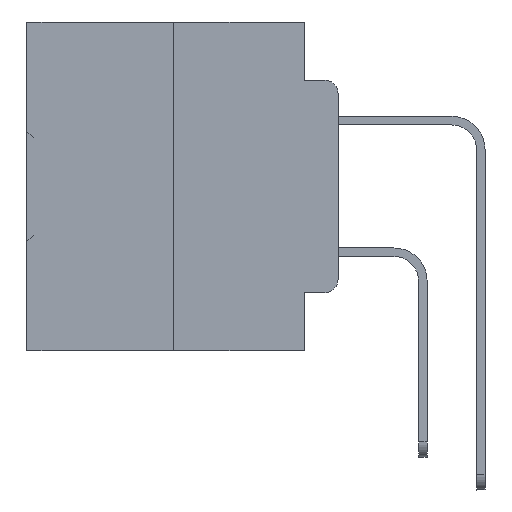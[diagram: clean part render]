
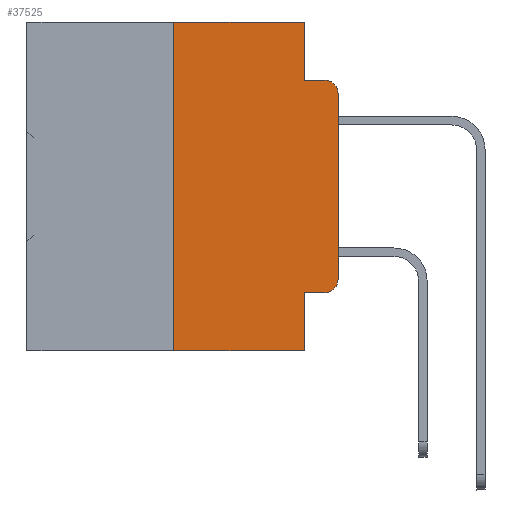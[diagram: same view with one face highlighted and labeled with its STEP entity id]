
A CAD part, left-side view. The second image highlights one B-rep face of the part: STEP entity #37525.
In plain terms, the highlighted planar face has unit normal (-1, 0, 0).
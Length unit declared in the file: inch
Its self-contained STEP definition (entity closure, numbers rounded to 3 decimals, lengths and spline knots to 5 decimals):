
#117 = CARTESIAN_POINT ( 'NONE',  ( 0., 0., 0. ) ) ;
#535 = VECTOR ( 'NONE', #15275, 39.37008 ) ;
#956 = LINE ( 'NONE', #13069, #31611 ) ;
#3079 = EDGE_CURVE ( 'NONE', #16572, #5358, #27038, .T. ) ;
#3636 = CARTESIAN_POINT ( 'NONE',  ( 0., 0., -0.3915 ) ) ;
#3899 = LINE ( 'NONE', #30909, #35743 ) ;
#4125 = VECTOR ( 'NONE', #36129, 39.37008 ) ;
#4657 = AXIS2_PLACEMENT_3D ( 'NONE', #34686, #34481, #37277 ) ;
#4710 = CARTESIAN_POINT ( 'NONE',  ( 0., 0.051, 0. ) ) ;
#5015 = VECTOR ( 'NONE', #21404, 39.37008 ) ;
#5358 = VERTEX_POINT ( 'NONE', #11432 ) ;
#5537 = ORIENTED_EDGE ( 'NONE', *, *, #33857, .T. ) ;
#5657 = DIRECTION ( 'NONE',  ( 0., 0., -1. ) ) ;
#6123 = CARTESIAN_POINT ( 'NONE',  ( 0., 0.02, -0.3915 ) ) ;
#6452 = LINE ( 'NONE', #27904, #19337 ) ;
#6461 = EDGE_CURVE ( 'NONE', #30614, #5358, #3899, .T. ) ;
#6745 = EDGE_LOOP ( 'NONE', ( #17902, #28723, #25407, #38897, #36173, #13882, #8554, #31702, #5537, #11947 ) ) ;
#8105 = VERTEX_POINT ( 'NONE', #12089 ) ;
#8540 = LINE ( 'NONE', #27211, #4125 ) ;
#8554 = ORIENTED_EDGE ( 'NONE', *, *, #3079, .T. ) ;
#8773 = CARTESIAN_POINT ( 'NONE',  ( 0., 0.473, -0.5 ) ) ;
#8885 = AXIS2_PLACEMENT_3D ( 'NONE', #6123, #9105, #9894 ) ;
#9071 = LINE ( 'NONE', #117, #5015 ) ;
#9105 = DIRECTION ( 'NONE',  ( -1., 0., 0. ) ) ;
#9532 = CARTESIAN_POINT ( 'NONE',  ( 0., 0.051, -0.4115 ) ) ;
#9894 = DIRECTION ( 'NONE',  ( 0., 0., -1. ) ) ;
#10096 = PLANE ( 'NONE',  #4657 ) ;
#11013 = VECTOR ( 'NONE', #23859, 39.37008 ) ;
#11432 = CARTESIAN_POINT ( 'NONE',  ( 0., 0.051, -0.5 ) ) ;
#11947 = ORIENTED_EDGE ( 'NONE', *, *, #22351, .T. ) ;
#12089 = CARTESIAN_POINT ( 'NONE',  ( 0., 0.02, -0.0885 ) ) ;
#12288 = LINE ( 'NONE', #15074, #19608 ) ;
#13069 = CARTESIAN_POINT ( 'NONE',  ( 0., 0.051, 0. ) ) ;
#13882 = ORIENTED_EDGE ( 'NONE', *, *, #33810, .F. ) ;
#14794 = CARTESIAN_POINT ( 'NONE',  ( 0., 0.02, -0.4115 ) ) ;
#15074 = CARTESIAN_POINT ( 'NONE',  ( 0., 0.25, 0. ) ) ;
#15275 = DIRECTION ( 'NONE',  ( 0., -1., 0. ) ) ;
#15579 = DIRECTION ( 'NONE',  ( 0., -1., 0. ) ) ;
#16572 = VERTEX_POINT ( 'NONE', #26756 ) ;
#17902 = ORIENTED_EDGE ( 'NONE', *, *, #34277, .T. ) ;
#18751 = CARTESIAN_POINT ( 'NONE',  ( 0., 0.051, -0.4115 ) ) ;
#19337 = VECTOR ( 'NONE', #15579, 39.37008 ) ;
#19608 = VECTOR ( 'NONE', #21645, 39.37008 ) ;
#21342 = DIRECTION ( 'NONE',  ( -1., 0., 0. ) ) ;
#21404 = DIRECTION ( 'NONE',  ( 0., 0., 1. ) ) ;
#21415 = DIRECTION ( 'NONE',  ( 0., 0., -1. ) ) ;
#21645 = DIRECTION ( 'NONE',  ( 0., 0., 1. ) ) ;
#22351 = EDGE_CURVE ( 'NONE', #37215, #22825, #36770, .T. ) ;
#22825 = VERTEX_POINT ( 'NONE', #3636 ) ;
#23859 = DIRECTION ( 'NONE',  ( 0., -1., 0. ) ) ;
#25192 = DIRECTION ( 'NONE',  ( 0., 0., -1. ) ) ;
#25407 = ORIENTED_EDGE ( 'NONE', *, *, #30808, .F. ) ;
#25988 = EDGE_CURVE ( 'NONE', #37928, #8105, #37871, .T. ) ;
#26674 = EDGE_CURVE ( 'NONE', #33964, #38569, #956, .T. ) ;
#26756 = CARTESIAN_POINT ( 'NONE',  ( 0., 0.25, -0.5 ) ) ;
#27038 = LINE ( 'NONE', #8773, #11013 ) ;
#27211 = CARTESIAN_POINT ( 'NONE',  ( 0., 0.051, -0.0885 ) ) ;
#27291 = CARTESIAN_POINT ( 'NONE',  ( 0., 0.02, -0.1085 ) ) ;
#27783 = LINE ( 'NONE', #9532, #535 ) ;
#27849 = VERTEX_POINT ( 'NONE', #30164 ) ;
#27904 = CARTESIAN_POINT ( 'NONE',  ( 0., 0.473, 0. ) ) ;
#28640 = CARTESIAN_POINT ( 'NONE',  ( 0., 0.051, -0.0885 ) ) ;
#28723 = ORIENTED_EDGE ( 'NONE', *, *, #25988, .T. ) ;
#30164 = CARTESIAN_POINT ( 'NONE',  ( 0., 0.25, 0. ) ) ;
#30614 = VERTEX_POINT ( 'NONE', #18751 ) ;
#30808 = EDGE_CURVE ( 'NONE', #38569, #8105, #8540, .T. ) ;
#30909 = CARTESIAN_POINT ( 'NONE',  ( 0., 0.051, 0. ) ) ;
#30935 = FACE_OUTER_BOUND ( 'NONE', #6745, .T. ) ;
#31611 = VECTOR ( 'NONE', #25192, 39.37008 ) ;
#31702 = ORIENTED_EDGE ( 'NONE', *, *, #6461, .F. ) ;
#33810 = EDGE_CURVE ( 'NONE', #16572, #27849, #12288, .T. ) ;
#33857 = EDGE_CURVE ( 'NONE', #30614, #37215, #27783, .T. ) ;
#33964 = VERTEX_POINT ( 'NONE', #4710 ) ;
#34252 = CARTESIAN_POINT ( 'NONE',  ( 0., 0., -0.1085 ) ) ;
#34277 = EDGE_CURVE ( 'NONE', #22825, #37928, #9071, .T. ) ;
#34481 = DIRECTION ( 'NONE',  ( 1., 0., 0. ) ) ;
#34686 = CARTESIAN_POINT ( 'NONE',  ( 0., 0.473, 0. ) ) ;
#35347 = AXIS2_PLACEMENT_3D ( 'NONE', #27291, #21342, #5657 ) ;
#35743 = VECTOR ( 'NONE', #21415, 39.37008 ) ;
#36129 = DIRECTION ( 'NONE',  ( 0., -1., 0. ) ) ;
#36163 = EDGE_CURVE ( 'NONE', #27849, #33964, #6452, .T. ) ;
#36173 = ORIENTED_EDGE ( 'NONE', *, *, #36163, .F. ) ;
#36770 = CIRCLE ( 'NONE', #8885, 0.02 ) ;
#37215 = VERTEX_POINT ( 'NONE', #14794 ) ;
#37277 = DIRECTION ( 'NONE',  ( 0., 0., -1. ) ) ;
#37525 = ADVANCED_FACE ( 'NONE', ( #30935 ), #10096, .F. ) ;
#37871 = CIRCLE ( 'NONE', #35347, 0.02 ) ;
#37928 = VERTEX_POINT ( 'NONE', #34252 ) ;
#38569 = VERTEX_POINT ( 'NONE', #28640 ) ;
#38897 = ORIENTED_EDGE ( 'NONE', *, *, #26674, .F. ) ;
